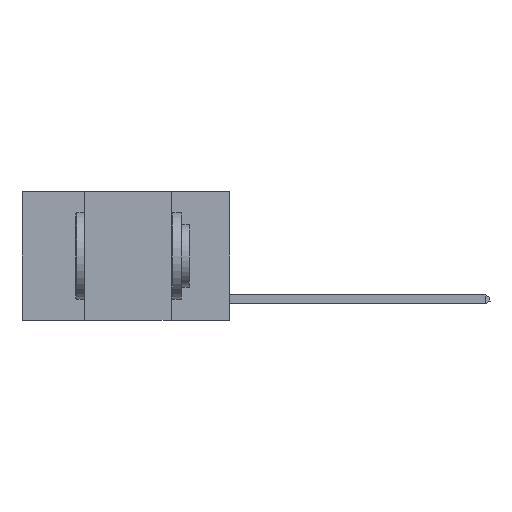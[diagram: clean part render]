
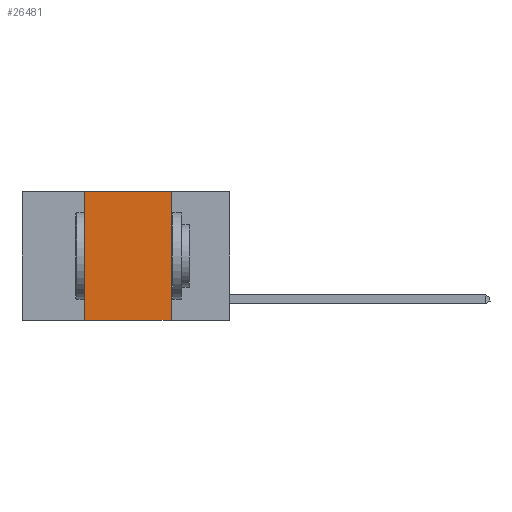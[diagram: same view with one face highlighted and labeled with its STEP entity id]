
A CAD part, left-side view. The second image highlights one B-rep face of the part: STEP entity #26481.
In plain terms, the highlighted planar face has unit normal (-1, 0, 0).
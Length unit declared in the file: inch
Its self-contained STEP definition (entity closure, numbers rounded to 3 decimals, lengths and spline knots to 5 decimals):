
#136 = DIRECTION ( 'NONE',  ( 0., 0., -1. ) ) ;
#494 = FACE_OUTER_BOUND ( 'NONE', #5394, .T. ) ;
#799 = VECTOR ( 'NONE', #7803, 39.37008 ) ;
#1048 = EDGE_CURVE ( 'NONE', #13477, #5269, #29260, .T. ) ;
#1912 = VECTOR ( 'NONE', #3853, 39.37008 ) ;
#2218 = VERTEX_POINT ( 'NONE', #21063 ) ;
#2391 = DIRECTION ( 'NONE',  ( 1., 0., 0. ) ) ;
#3853 = DIRECTION ( 'NONE',  ( 0., -1., 0. ) ) ;
#4430 = CARTESIAN_POINT ( 'NONE',  ( 0., 0.42, 0. ) ) ;
#5041 = AXIS2_PLACEMENT_3D ( 'NONE', #11940, #2391, #136 ) ;
#5269 = VERTEX_POINT ( 'NONE', #4430 ) ;
#5394 = EDGE_LOOP ( 'NONE', ( #12211, #30358, #24567, #6604 ) ) ;
#6604 = ORIENTED_EDGE ( 'NONE', *, *, #26856, .T. ) ;
#7803 = DIRECTION ( 'NONE',  ( 0., 0., -1. ) ) ;
#9898 = VECTOR ( 'NONE', #26863, 39.37008 ) ;
#11148 = VERTEX_POINT ( 'NONE', #19099 ) ;
#11940 = CARTESIAN_POINT ( 'NONE',  ( 0., 0.6, 0. ) ) ;
#12055 = CARTESIAN_POINT ( 'NONE',  ( 0., 0.42, -0.37 ) ) ;
#12211 = ORIENTED_EDGE ( 'NONE', *, *, #14050, .F. ) ;
#13423 = LINE ( 'NONE', #15168, #799 ) ;
#13477 = VERTEX_POINT ( 'NONE', #12055 ) ;
#14050 = EDGE_CURVE ( 'NONE', #11148, #2218, #13423, .T. ) ;
#14364 = PLANE ( 'NONE',  #5041 ) ;
#14717 = LINE ( 'NONE', #24332, #9898 ) ;
#15168 = CARTESIAN_POINT ( 'NONE',  ( 0., 0.17, 0. ) ) ;
#19099 = CARTESIAN_POINT ( 'NONE',  ( 0., 0.17, 0. ) ) ;
#21063 = CARTESIAN_POINT ( 'NONE',  ( 0., 0.17, -0.37 ) ) ;
#21284 = LINE ( 'NONE', #27823, #1912 ) ;
#23675 = DIRECTION ( 'NONE',  ( 0., 0., 1. ) ) ;
#24332 = CARTESIAN_POINT ( 'NONE',  ( 0., 0.6, 0. ) ) ;
#24567 = ORIENTED_EDGE ( 'NONE', *, *, #1048, .F. ) ;
#25299 = EDGE_CURVE ( 'NONE', #5269, #11148, #14717, .T. ) ;
#26289 = CARTESIAN_POINT ( 'NONE',  ( 0., 0.42, 0. ) ) ;
#26481 = ADVANCED_FACE ( 'NONE', ( #494 ), #14364, .F. ) ;
#26856 = EDGE_CURVE ( 'NONE', #13477, #2218, #21284, .T. ) ;
#26863 = DIRECTION ( 'NONE',  ( 0., -1., 0. ) ) ;
#27823 = CARTESIAN_POINT ( 'NONE',  ( 0., 0.6, -0.37 ) ) ;
#28521 = VECTOR ( 'NONE', #23675, 39.37008 ) ;
#29260 = LINE ( 'NONE', #26289, #28521 ) ;
#30358 = ORIENTED_EDGE ( 'NONE', *, *, #25299, .F. ) ;
